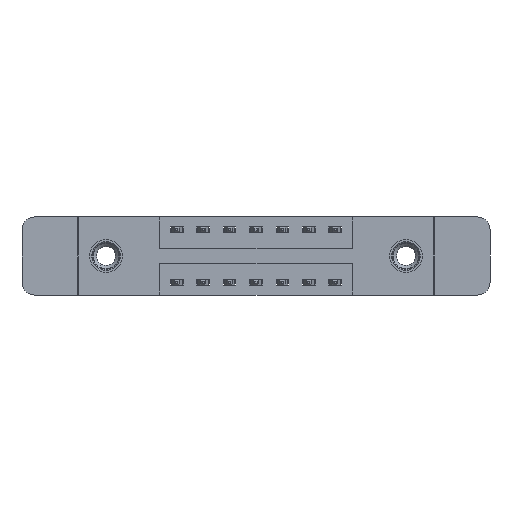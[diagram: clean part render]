
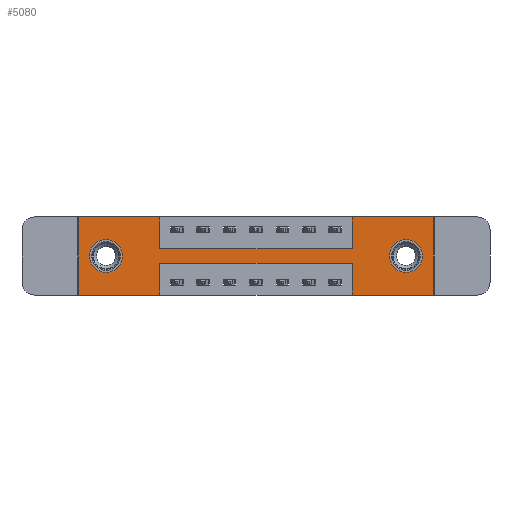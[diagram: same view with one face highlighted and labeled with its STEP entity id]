
A CAD part, front view. The second image highlights one B-rep face of the part: STEP entity #5080.
In plain terms, the highlighted planar face has unit normal (0, -1, 0).
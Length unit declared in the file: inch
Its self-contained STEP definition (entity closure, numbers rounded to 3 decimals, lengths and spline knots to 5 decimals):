
#184 = ORIENTED_EDGE ( 'NONE', *, *, #2247, .F. ) ;
#217 = ORIENTED_EDGE ( 'NONE', *, *, #5778, .T. ) ;
#260 = CARTESIAN_POINT ( 'NONE',  ( 0., 0., -0.37 ) ) ;
#333 = CARTESIAN_POINT ( 'NONE',  ( 0., 0., -0.37 ) ) ;
#408 = VECTOR ( 'NONE', #10305, 39.37008 ) ;
#462 = ORIENTED_EDGE ( 'NONE', *, *, #12987, .F. ) ;
#476 = CARTESIAN_POINT ( 'NONE',  ( 0.1325, 0., -0.185 ) ) ;
#534 = VERTEX_POINT ( 'NONE', #10536 ) ;
#619 = DIRECTION ( 'NONE',  ( 0., 0., -1. ) ) ;
#808 = VECTOR ( 'NONE', #6077, 39.37008 ) ;
#815 = DIRECTION ( 'NONE',  ( 0., 0., -1. ) ) ;
#884 = AXIS2_PLACEMENT_3D ( 'NONE', #476, #3842, #4955 ) ;
#943 = EDGE_CURVE ( 'NONE', #11170, #14355, #5869, .T. ) ;
#976 = CARTESIAN_POINT ( 'NONE',  ( 0., 0., -0.37 ) ) ;
#979 = VECTOR ( 'NONE', #5774, 39.37008 ) ;
#1044 = VERTEX_POINT ( 'NONE', #9888 ) ;
#1063 = EDGE_CURVE ( 'NONE', #9326, #12095, #7108, .T. ) ;
#1790 = PLANE ( 'NONE',  #7636 ) ;
#1950 = DIRECTION ( 'NONE',  ( 0., 0., 1. ) ) ;
#2028 = DIRECTION ( 'NONE',  ( 0., 1., 0. ) ) ;
#2048 = VECTOR ( 'NONE', #12814, 39.37008 ) ;
#2051 = EDGE_CURVE ( 'NONE', #5903, #8560, #3382, .T. ) ;
#2247 = EDGE_CURVE ( 'NONE', #5238, #9326, #10721, .T. ) ;
#2269 = ORIENTED_EDGE ( 'NONE', *, *, #9768, .F. ) ;
#2758 = CARTESIAN_POINT ( 'NONE',  ( 0.1325, 0., -0.107 ) ) ;
#2821 = CARTESIAN_POINT ( 'NONE',  ( 1.5525, 0., -0.263 ) ) ;
#2952 = DIRECTION ( 'NONE',  ( 0., 0., 1. ) ) ;
#2957 = ORIENTED_EDGE ( 'NONE', *, *, #3465, .F. ) ;
#2967 = ORIENTED_EDGE ( 'NONE', *, *, #1063, .F. ) ;
#3264 = DIRECTION ( 'NONE',  ( 1., 0., 0. ) ) ;
#3382 = CIRCLE ( 'NONE', #7577, 0.078 ) ;
#3412 = VERTEX_POINT ( 'NONE', #6377 ) ;
#3465 = EDGE_CURVE ( 'NONE', #9264, #8039, #7218, .T. ) ;
#3842 = DIRECTION ( 'NONE',  ( 0., 1., 0. ) ) ;
#3869 = ORIENTED_EDGE ( 'NONE', *, *, #2051, .T. ) ;
#3874 = VECTOR ( 'NONE', #7243, 39.37008 ) ;
#3881 = LINE ( 'NONE', #260, #408 ) ;
#4135 = ORIENTED_EDGE ( 'NONE', *, *, #7315, .T. ) ;
#4179 = ORIENTED_EDGE ( 'NONE', *, *, #4561, .F. ) ;
#4234 = VECTOR ( 'NONE', #5932, 39.37008 ) ;
#4515 = ORIENTED_EDGE ( 'NONE', *, *, #14009, .F. ) ;
#4561 = EDGE_CURVE ( 'NONE', #3412, #9444, #7233, .T. ) ;
#4773 = VECTOR ( 'NONE', #3264, 39.37008 ) ;
#4927 = CARTESIAN_POINT ( 'NONE',  ( 1.2975, 0., 0. ) ) ;
#4936 = CARTESIAN_POINT ( 'NONE',  ( 0.3875, 0., -0.22 ) ) ;
#4955 = DIRECTION ( 'NONE',  ( 0., 0., 1. ) ) ;
#5080 = ADVANCED_FACE ( 'NONE', ( #10859, #11570, #10499 ), #1790, .T. ) ;
#5123 = CARTESIAN_POINT ( 'NONE',  ( 1.5525, 0., -0.185 ) ) ;
#5238 = VERTEX_POINT ( 'NONE', #8555 ) ;
#5397 = ORIENTED_EDGE ( 'NONE', *, *, #13572, .T. ) ;
#5431 = CARTESIAN_POINT ( 'NONE',  ( 1.2975, 0., -0.37 ) ) ;
#5500 = LINE ( 'NONE', #10932, #14273 ) ;
#5528 = LINE ( 'NONE', #4936, #2048 ) ;
#5774 = DIRECTION ( 'NONE',  ( 0., 0., 1. ) ) ;
#5778 = EDGE_CURVE ( 'NONE', #1044, #12205, #13450, .T. ) ;
#5869 = LINE ( 'NONE', #4927, #12725 ) ;
#5903 = VERTEX_POINT ( 'NONE', #9469 ) ;
#5932 = DIRECTION ( 'NONE',  ( -1., 0., 0. ) ) ;
#6075 = DIRECTION ( 'NONE',  ( 0., 0., 1. ) ) ;
#6077 = DIRECTION ( 'NONE',  ( 0., 0., -1. ) ) ;
#6134 = LINE ( 'NONE', #7498, #14160 ) ;
#6377 = CARTESIAN_POINT ( 'NONE',  ( 0.3875, 0., -0.22 ) ) ;
#6547 = CARTESIAN_POINT ( 'NONE',  ( 0., 0., 0. ) ) ;
#6644 = CARTESIAN_POINT ( 'NONE',  ( 0.3875, 0., -0.15 ) ) ;
#6891 = CARTESIAN_POINT ( 'NONE',  ( 0.3875, 0., -0.37 ) ) ;
#7108 = LINE ( 'NONE', #12004, #808 ) ;
#7111 = CARTESIAN_POINT ( 'NONE',  ( 1.685, 0., -0.37 ) ) ;
#7218 = LINE ( 'NONE', #333, #4234 ) ;
#7232 = CARTESIAN_POINT ( 'NONE',  ( 0.3875, 0., -0.15 ) ) ;
#7233 = LINE ( 'NONE', #10648, #3874 ) ;
#7243 = DIRECTION ( 'NONE',  ( 0., 0., -1. ) ) ;
#7315 = EDGE_CURVE ( 'NONE', #12205, #1044, #9956, .T. ) ;
#7498 = CARTESIAN_POINT ( 'NONE',  ( 1.685, 0., 0. ) ) ;
#7577 = AXIS2_PLACEMENT_3D ( 'NONE', #5123, #9549, #815 ) ;
#7630 = ORIENTED_EDGE ( 'NONE', *, *, #12145, .F. ) ;
#7636 = AXIS2_PLACEMENT_3D ( 'NONE', #976, #11901, #619 ) ;
#7672 = VERTEX_POINT ( 'NONE', #8591 ) ;
#7788 = AXIS2_PLACEMENT_3D ( 'NONE', #8875, #2028, #14407 ) ;
#8039 = VERTEX_POINT ( 'NONE', #5431 ) ;
#8120 = AXIS2_PLACEMENT_3D ( 'NONE', #8517, #9643, #2952 ) ;
#8248 = DIRECTION ( 'NONE',  ( 1., 0., 0. ) ) ;
#8517 = CARTESIAN_POINT ( 'NONE',  ( 0.1325, 0., -0.185 ) ) ;
#8555 = CARTESIAN_POINT ( 'NONE',  ( 0., 0., 0. ) ) ;
#8560 = VERTEX_POINT ( 'NONE', #2821 ) ;
#8591 = CARTESIAN_POINT ( 'NONE',  ( 0., 0., -0.37 ) ) ;
#8654 = ORIENTED_EDGE ( 'NONE', *, *, #943, .F. ) ;
#8841 = CARTESIAN_POINT ( 'NONE',  ( 0., 0., 0. ) ) ;
#8875 = CARTESIAN_POINT ( 'NONE',  ( 1.5525, 0., -0.185 ) ) ;
#9191 = CARTESIAN_POINT ( 'NONE',  ( 1.2975, 0., -0.22 ) ) ;
#9264 = VERTEX_POINT ( 'NONE', #7111 ) ;
#9326 = VERTEX_POINT ( 'NONE', #13951 ) ;
#9358 = LINE ( 'NONE', #13690, #979 ) ;
#9444 = VERTEX_POINT ( 'NONE', #6891 ) ;
#9469 = CARTESIAN_POINT ( 'NONE',  ( 1.5525, 0., -0.107 ) ) ;
#9470 = DIRECTION ( 'NONE',  ( 1., 0., 0. ) ) ;
#9549 = DIRECTION ( 'NONE',  ( 0., 1., 0. ) ) ;
#9568 = CARTESIAN_POINT ( 'NONE',  ( 1.2975, 0., 0. ) ) ;
#9643 = DIRECTION ( 'NONE',  ( 0., 1., 0. ) ) ;
#9768 = EDGE_CURVE ( 'NONE', #12095, #11170, #10156, .T. ) ;
#9888 = CARTESIAN_POINT ( 'NONE',  ( 0.1325, 0., -0.263 ) ) ;
#9956 = CIRCLE ( 'NONE', #8120, 0.078 ) ;
#10156 = LINE ( 'NONE', #6644, #13011 ) ;
#10305 = DIRECTION ( 'NONE',  ( -1., 0., 0. ) ) ;
#10499 = FACE_OUTER_BOUND ( 'NONE', #11848, .T. ) ;
#10520 = EDGE_CURVE ( 'NONE', #534, #9264, #6134, .T. ) ;
#10536 = CARTESIAN_POINT ( 'NONE',  ( 1.685, 0., 0. ) ) ;
#10648 = CARTESIAN_POINT ( 'NONE',  ( 0.3875, 0., -0.37 ) ) ;
#10721 = LINE ( 'NONE', #8841, #4773 ) ;
#10785 = DIRECTION ( 'NONE',  ( 0., 0., -1. ) ) ;
#10859 = FACE_BOUND ( 'NONE', #10938, .T. ) ;
#10932 = CARTESIAN_POINT ( 'NONE',  ( 0., 0., 0. ) ) ;
#10938 = EDGE_LOOP ( 'NONE', ( #3869, #5397 ) ) ;
#11170 = VERTEX_POINT ( 'NONE', #11662 ) ;
#11243 = EDGE_CURVE ( 'NONE', #13015, #3412, #5528, .T. ) ;
#11570 = FACE_BOUND ( 'NONE', #13149, .T. ) ;
#11662 = CARTESIAN_POINT ( 'NONE',  ( 1.2975, 0., -0.15 ) ) ;
#11792 = ORIENTED_EDGE ( 'NONE', *, *, #10520, .F. ) ;
#11848 = EDGE_LOOP ( 'NONE', ( #4179, #12376, #462, #2957, #11792, #7630, #8654, #2269, #2967, #184, #4515, #13402 ) ) ;
#11901 = DIRECTION ( 'NONE',  ( 0., -1., 0. ) ) ;
#12004 = CARTESIAN_POINT ( 'NONE',  ( 0.3875, 0., 0. ) ) ;
#12095 = VERTEX_POINT ( 'NONE', #7232 ) ;
#12145 = EDGE_CURVE ( 'NONE', #14355, #534, #5500, .T. ) ;
#12205 = VERTEX_POINT ( 'NONE', #2758 ) ;
#12329 = LINE ( 'NONE', #6547, #12703 ) ;
#12376 = ORIENTED_EDGE ( 'NONE', *, *, #11243, .F. ) ;
#12703 = VECTOR ( 'NONE', #1950, 39.37008 ) ;
#12725 = VECTOR ( 'NONE', #6075, 39.37008 ) ;
#12814 = DIRECTION ( 'NONE',  ( -1., 0., 0. ) ) ;
#12987 = EDGE_CURVE ( 'NONE', #8039, #13015, #9358, .T. ) ;
#13011 = VECTOR ( 'NONE', #8248, 39.37008 ) ;
#13015 = VERTEX_POINT ( 'NONE', #9191 ) ;
#13045 = CIRCLE ( 'NONE', #7788, 0.078 ) ;
#13149 = EDGE_LOOP ( 'NONE', ( #4135, #217 ) ) ;
#13402 = ORIENTED_EDGE ( 'NONE', *, *, #14442, .F. ) ;
#13450 = CIRCLE ( 'NONE', #884, 0.078 ) ;
#13572 = EDGE_CURVE ( 'NONE', #8560, #5903, #13045, .T. ) ;
#13690 = CARTESIAN_POINT ( 'NONE',  ( 1.2975, 0., -0.37 ) ) ;
#13951 = CARTESIAN_POINT ( 'NONE',  ( 0.3875, 0., 0. ) ) ;
#14009 = EDGE_CURVE ( 'NONE', #7672, #5238, #12329, .T. ) ;
#14160 = VECTOR ( 'NONE', #10785, 39.37008 ) ;
#14273 = VECTOR ( 'NONE', #9470, 39.37008 ) ;
#14355 = VERTEX_POINT ( 'NONE', #9568 ) ;
#14407 = DIRECTION ( 'NONE',  ( 0., 0., -1. ) ) ;
#14442 = EDGE_CURVE ( 'NONE', #9444, #7672, #3881, .T. ) ;
